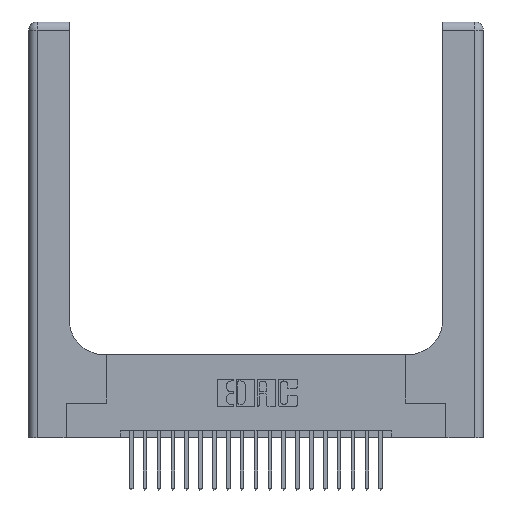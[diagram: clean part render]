
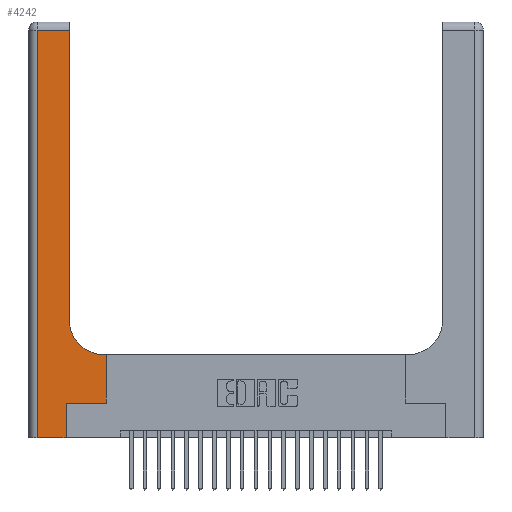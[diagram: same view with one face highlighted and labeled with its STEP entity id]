
A CAD part, top view. The second image highlights one B-rep face of the part: STEP entity #4242.
In plain terms, the highlighted planar face has unit normal (0, 0, 1).
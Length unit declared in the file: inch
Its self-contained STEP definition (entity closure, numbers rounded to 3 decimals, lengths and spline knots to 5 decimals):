
#142 = CARTESIAN_POINT ( 'NONE',  ( 0.269, 0.25, 0.37 ) ) ;
#725 = FACE_OUTER_BOUND ( 'NONE', #8444, .T. ) ;
#748 = ORIENTED_EDGE ( 'NONE', *, *, #22633, .T. ) ;
#1003 = ORIENTED_EDGE ( 'NONE', *, *, #9005, .T. ) ;
#1115 = CARTESIAN_POINT ( 'NONE',  ( 0.269, 0., 0.37 ) ) ;
#1271 = CARTESIAN_POINT ( 'NONE',  ( 0.5415, 0.6, 0.37 ) ) ;
#1334 = VECTOR ( 'NONE', #22862, 39.37008 ) ;
#1923 = DIRECTION ( 'NONE',  ( 0., 1., 0. ) ) ;
#1951 = VERTEX_POINT ( 'NONE', #17143 ) ;
#2205 = DIRECTION ( 'NONE',  ( 0., 0., -1. ) ) ;
#2593 = VERTEX_POINT ( 'NONE', #1271 ) ;
#4242 = ADVANCED_FACE ( 'NONE', ( #725 ), #11291, .F. ) ;
#4281 = EDGE_CURVE ( 'NONE', #2593, #11534, #18281, .T. ) ;
#4671 = VECTOR ( 'NONE', #9323, 39.37008 ) ;
#7152 = CARTESIAN_POINT ( 'NONE',  ( 0.269, 0., 0.37 ) ) ;
#7748 = CARTESIAN_POINT ( 'NONE',  ( 0.2915, 2.94, 0.37 ) ) ;
#8174 = EDGE_CURVE ( 'NONE', #1951, #20969, #14268, .T. ) ;
#8444 = EDGE_LOOP ( 'NONE', ( #748, #11080, #21548, #1003, #12436, #8707, #15781, #18018, #13257 ) ) ;
#8595 = EDGE_CURVE ( 'NONE', #15076, #2593, #15254, .T. ) ;
#8689 = EDGE_CURVE ( 'NONE', #15510, #1951, #8805, .T. ) ;
#8707 = ORIENTED_EDGE ( 'NONE', *, *, #8174, .T. ) ;
#8805 = LINE ( 'NONE', #7152, #17749 ) ;
#9005 = EDGE_CURVE ( 'NONE', #21309, #15510, #22622, .T. ) ;
#9323 = DIRECTION ( 'NONE',  ( 1., 0., 0. ) ) ;
#9506 = DIRECTION ( 'NONE',  ( -1., 0., 0. ) ) ;
#9645 = DIRECTION ( 'NONE',  ( 0., 0., -1. ) ) ;
#9997 = CARTESIAN_POINT ( 'NONE',  ( 0.06, 2.94, 0.37 ) ) ;
#10124 = VECTOR ( 'NONE', #10401, 39.37008 ) ;
#10401 = DIRECTION ( 'NONE',  ( 0., 1., 0. ) ) ;
#10560 = CARTESIAN_POINT ( 'NONE',  ( 0.2915, 0.6, 0.37 ) ) ;
#11080 = ORIENTED_EDGE ( 'NONE', *, *, #21722, .T. ) ;
#11123 = VERTEX_POINT ( 'NONE', #7748 ) ;
#11291 = PLANE ( 'NONE',  #16429 ) ;
#11534 = VERTEX_POINT ( 'NONE', #15941 ) ;
#11652 = CARTESIAN_POINT ( 'NONE',  ( 0.5585, 0.25, 0.37 ) ) ;
#11891 = EDGE_CURVE ( 'NONE', #20969, #15076, #16545, .T. ) ;
#12205 = CARTESIAN_POINT ( 'NONE',  ( 0.2915, 3., 0.37 ) ) ;
#12436 = ORIENTED_EDGE ( 'NONE', *, *, #8689, .T. ) ;
#13123 = CARTESIAN_POINT ( 'NONE',  ( 0., 3., 0.37 ) ) ;
#13257 = ORIENTED_EDGE ( 'NONE', *, *, #4281, .T. ) ;
#13687 = CARTESIAN_POINT ( 'NONE',  ( 0., 0., 0.37 ) ) ;
#14190 = LINE ( 'NONE', #15289, #18342 ) ;
#14268 = LINE ( 'NONE', #142, #4671 ) ;
#14442 = CARTESIAN_POINT ( 'NONE',  ( 0.5585, 0.6, 0.37 ) ) ;
#14706 = EDGE_CURVE ( 'NONE', #17744, #21309, #14190, .T. ) ;
#14876 = LINE ( 'NONE', #12205, #10124 ) ;
#14881 = DIRECTION ( 'NONE',  ( -1., 0., 0. ) ) ;
#15076 = VERTEX_POINT ( 'NONE', #14442 ) ;
#15254 = LINE ( 'NONE', #10560, #1334 ) ;
#15289 = CARTESIAN_POINT ( 'NONE',  ( 0.06, 3., 0.37 ) ) ;
#15510 = VERTEX_POINT ( 'NONE', #1115 ) ;
#15781 = ORIENTED_EDGE ( 'NONE', *, *, #11891, .T. ) ;
#15941 = CARTESIAN_POINT ( 'NONE',  ( 0.2915, 0.85, 0.37 ) ) ;
#16354 = VECTOR ( 'NONE', #22412, 39.37008 ) ;
#16429 = AXIS2_PLACEMENT_3D ( 'NONE', #13123, #2205, #14881 ) ;
#16545 = LINE ( 'NONE', #11652, #20625 ) ;
#17032 = DIRECTION ( 'NONE',  ( 0., 1., 0. ) ) ;
#17143 = CARTESIAN_POINT ( 'NONE',  ( 0.269, 0.25, 0.37 ) ) ;
#17609 = AXIS2_PLACEMENT_3D ( 'NONE', #20236, #9645, #21991 ) ;
#17744 = VERTEX_POINT ( 'NONE', #9997 ) ;
#17749 = VECTOR ( 'NONE', #1923, 39.37008 ) ;
#17963 = LINE ( 'NONE', #20097, #18532 ) ;
#18018 = ORIENTED_EDGE ( 'NONE', *, *, #8595, .T. ) ;
#18281 = CIRCLE ( 'NONE', #17609, 0.25 ) ;
#18342 = VECTOR ( 'NONE', #22246, 39.37008 ) ;
#18532 = VECTOR ( 'NONE', #9506, 39.37008 ) ;
#19893 = CARTESIAN_POINT ( 'NONE',  ( 0.5585, 0.25, 0.37 ) ) ;
#20097 = CARTESIAN_POINT ( 'NONE',  ( 0., 2.94, 0.37 ) ) ;
#20236 = CARTESIAN_POINT ( 'NONE',  ( 0.5415, 0.85, 0.37 ) ) ;
#20625 = VECTOR ( 'NONE', #17032, 39.37008 ) ;
#20969 = VERTEX_POINT ( 'NONE', #19893 ) ;
#21309 = VERTEX_POINT ( 'NONE', #22393 ) ;
#21548 = ORIENTED_EDGE ( 'NONE', *, *, #14706, .T. ) ;
#21722 = EDGE_CURVE ( 'NONE', #11123, #17744, #17963, .T. ) ;
#21991 = DIRECTION ( 'NONE',  ( 1., 0., 0. ) ) ;
#22246 = DIRECTION ( 'NONE',  ( 0., -1., 0. ) ) ;
#22393 = CARTESIAN_POINT ( 'NONE',  ( 0.06, 0., 0.37 ) ) ;
#22412 = DIRECTION ( 'NONE',  ( 1., 0., 0. ) ) ;
#22622 = LINE ( 'NONE', #13687, #16354 ) ;
#22633 = EDGE_CURVE ( 'NONE', #11534, #11123, #14876, .T. ) ;
#22862 = DIRECTION ( 'NONE',  ( -1., 0., 0. ) ) ;
